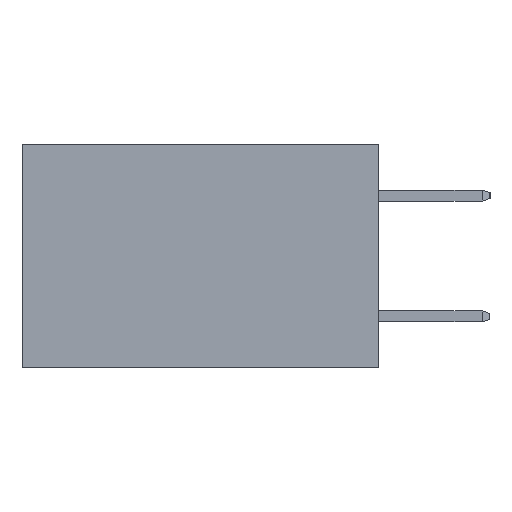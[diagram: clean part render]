
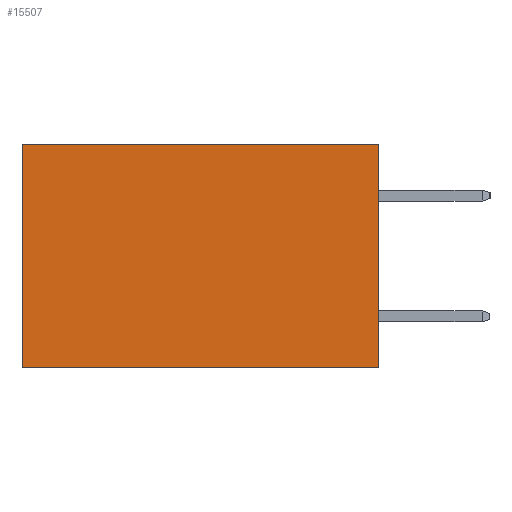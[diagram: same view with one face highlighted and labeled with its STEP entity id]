
A CAD part, left-side view. The second image highlights one B-rep face of the part: STEP entity #15507.
In plain terms, the highlighted planar face has unit normal (-1, 0, 0).
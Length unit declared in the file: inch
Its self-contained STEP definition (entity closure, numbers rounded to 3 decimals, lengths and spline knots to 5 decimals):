
#1378 = VECTOR ( 'NONE', #14839, 39.37008 ) ;
#1860 = LINE ( 'NONE', #4806, #15043 ) ;
#2287 = ORIENTED_EDGE ( 'NONE', *, *, #15136, .F. ) ;
#2868 = EDGE_CURVE ( 'NONE', #6532, #3970, #15143, .T. ) ;
#3342 = CARTESIAN_POINT ( 'NONE',  ( 0.277, 0., 0. ) ) ;
#3430 = EDGE_CURVE ( 'NONE', #3970, #9320, #21070, .T. ) ;
#3558 = FACE_OUTER_BOUND ( 'NONE', #6447, .T. ) ;
#3970 = VERTEX_POINT ( 'NONE', #15564 ) ;
#4806 = CARTESIAN_POINT ( 'NONE',  ( 0.277, 0., -0.37 ) ) ;
#6020 = CARTESIAN_POINT ( 'NONE',  ( 0.277, 0., -0.37 ) ) ;
#6367 = CARTESIAN_POINT ( 'NONE',  ( 0.277, 0.59, -0.37 ) ) ;
#6447 = EDGE_LOOP ( 'NONE', ( #15434, #19829, #2287, #7515 ) ) ;
#6532 = VERTEX_POINT ( 'NONE', #3342 ) ;
#6536 = DIRECTION ( 'NONE',  ( 0., 0., -1. ) ) ;
#7515 = ORIENTED_EDGE ( 'NONE', *, *, #2868, .T. ) ;
#7681 = DIRECTION ( 'NONE',  ( 0., 0., -1. ) ) ;
#8760 = VECTOR ( 'NONE', #20984, 39.37008 ) ;
#9320 = VERTEX_POINT ( 'NONE', #6367 ) ;
#10987 = PLANE ( 'NONE',  #20692 ) ;
#11892 = VERTEX_POINT ( 'NONE', #20254 ) ;
#13593 = DIRECTION ( 'NONE',  ( 0., 0., -1. ) ) ;
#14002 = EDGE_CURVE ( 'NONE', #11892, #9320, #19474, .T. ) ;
#14839 = DIRECTION ( 'NONE',  ( 0., 1., 0. ) ) ;
#15043 = VECTOR ( 'NONE', #6536, 39.37008 ) ;
#15136 = EDGE_CURVE ( 'NONE', #6532, #11892, #1860, .T. ) ;
#15143 = LINE ( 'NONE', #15510, #1378 ) ;
#15434 = ORIENTED_EDGE ( 'NONE', *, *, #3430, .T. ) ;
#15507 = ADVANCED_FACE ( 'NONE', ( #3558 ), #10987, .F. ) ;
#15510 = CARTESIAN_POINT ( 'NONE',  ( 0.277, 0., 0. ) ) ;
#15564 = CARTESIAN_POINT ( 'NONE',  ( 0.277, 0.59, 0. ) ) ;
#15972 = CARTESIAN_POINT ( 'NONE',  ( 0.277, 0., -0.37 ) ) ;
#16156 = CARTESIAN_POINT ( 'NONE',  ( 0.277, 0.59, -0.37 ) ) ;
#17752 = DIRECTION ( 'NONE',  ( 1., 0., 0. ) ) ;
#19474 = LINE ( 'NONE', #15972, #8760 ) ;
#19829 = ORIENTED_EDGE ( 'NONE', *, *, #14002, .F. ) ;
#20254 = CARTESIAN_POINT ( 'NONE',  ( 0.277, 0., -0.37 ) ) ;
#20553 = VECTOR ( 'NONE', #13593, 39.37008 ) ;
#20692 = AXIS2_PLACEMENT_3D ( 'NONE', #6020, #17752, #7681 ) ;
#20984 = DIRECTION ( 'NONE',  ( 0., 1., 0. ) ) ;
#21070 = LINE ( 'NONE', #16156, #20553 ) ;
